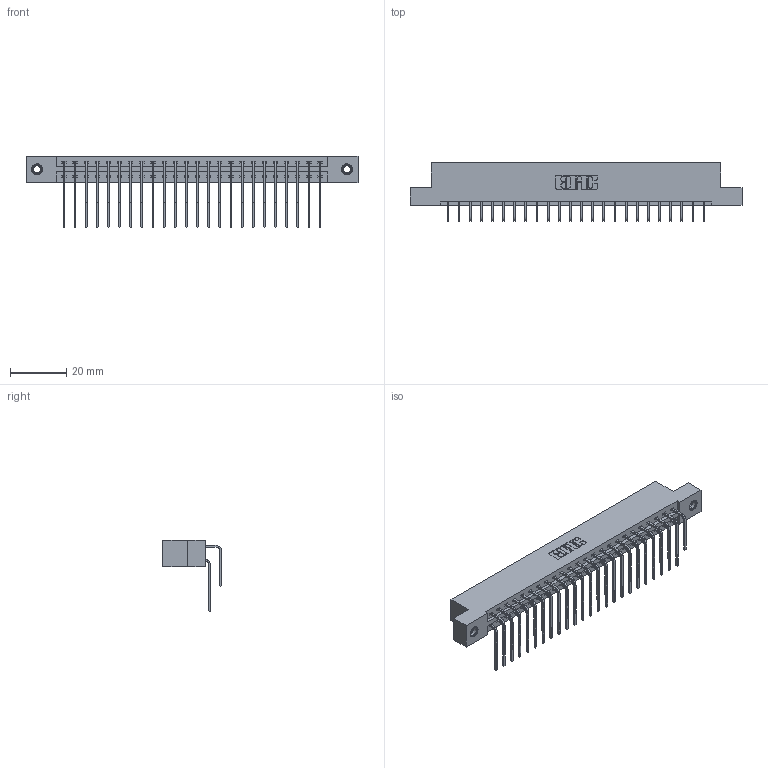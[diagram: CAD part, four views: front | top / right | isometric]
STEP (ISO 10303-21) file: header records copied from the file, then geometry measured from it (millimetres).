
FILE_DESCRIPTION (( 'STEP AP203' ), '1' );
FILE_NAME ('387-048-559-207.STEP', '2019-10-18T10:53:07', ( '' ), ( '' ), 'SwSTEP 2.0', 'SolidWorks 2016', '' );
FILE_SCHEMA (( 'CONFIG_CONTROL_DESIGN' ));
Length unit declared in the file: inch
Products named in the file (5): 337 Part_Flush Mounting Lugs - 0.156 Dia-TI; 345-292-001_559 Tail - 2; 345-292-001_558 559 Tail - 1; 387-048-559-207; 345-250-001_345-250-005-103
Assembly tree (51 placements, depth 2):
  387-048-559-207
    337 Part_Flush Mounting Lugs - 0.156 Dia-TI
    345-292-001_558 559 Tail - 1  x24
    345-292-001_559 Tail - 2  x24
    345-250-001_345-250-005-103  x2
Bounding box: 118.11 x 20.9 x 25.53 mm (x, y, z)
Volume: 12471.2 mm3; surface area: 15350.1 mm2
Topology: 51 solids, 51 shells, 2862 faces, 8463 edges, 5570 vertices
Faces by surface type: plane 2022, cylinder 824, cone 12, torus 4
Entity records: 23906 total; most frequent: CARTESIAN_POINT 4068, ORIENTED_EDGE 3946, DIRECTION 3507, EDGE_CURVE 1973, VECTOR 1785, LINE 1785, VERTEX_POINT 1308, AXIS2_PLACEMENT_3D 861
